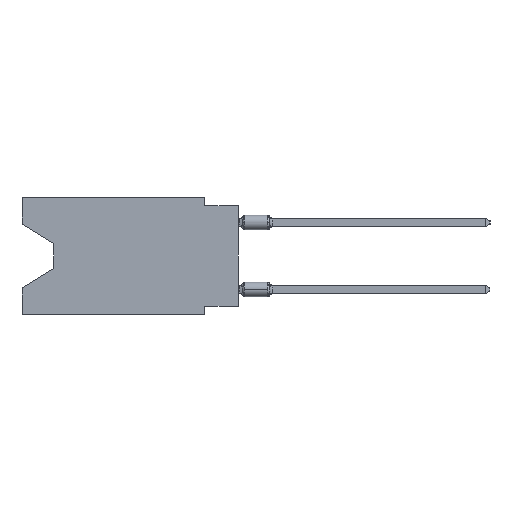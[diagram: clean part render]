
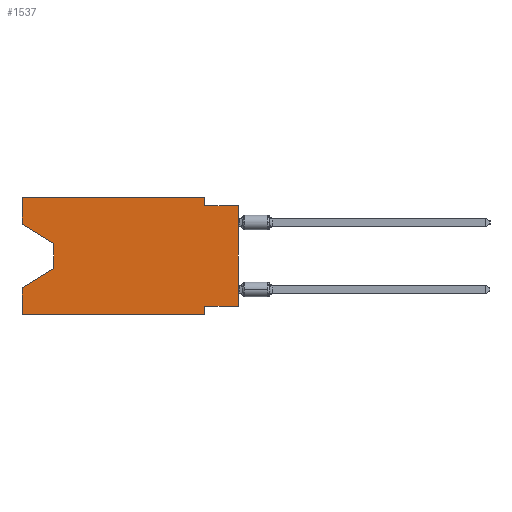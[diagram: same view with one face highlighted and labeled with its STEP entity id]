
A CAD part, left-side view. The second image highlights one B-rep face of the part: STEP entity #1537.
In plain terms, the highlighted planar face has unit normal (-1, 0, 0).
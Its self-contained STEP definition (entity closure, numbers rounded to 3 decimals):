
#347 = CARTESIAN_POINT ( 'NONE',  ( 0., 16.383, -6.852 ) ) ;
#589 = EDGE_CURVE ( 'NONE', #2754, #10713, #4848, .T. ) ;
#617 = LINE ( 'NONE', #11900, #15116 ) ;
#751 = ORIENTED_EDGE ( 'NONE', *, *, #9387, .F. ) ;
#971 = ORIENTED_EDGE ( 'NONE', *, *, #14238, .F. ) ;
#1141 = DIRECTION ( 'NONE',  ( 0., 0., -1. ) ) ;
#1215 = CARTESIAN_POINT ( 'NONE',  ( 0., 0., 0. ) ) ;
#1287 = VERTEX_POINT ( 'NONE', #16835 ) ;
#1289 = EDGE_CURVE ( 'NONE', #13922, #15580, #4266, .T. ) ;
#1366 = DIRECTION ( 'NONE',  ( 0., 0., 1. ) ) ;
#1431 = LINE ( 'NONE', #13906, #12771 ) ;
#1537 = ADVANCED_FACE ( 'NONE', ( #4064 ), #15334, .F. ) ;
#2052 = VERTEX_POINT ( 'NONE', #15244 ) ;
#2508 = DIRECTION ( 'NONE',  ( 1., 0., 0. ) ) ;
#2754 = VERTEX_POINT ( 'NONE', #2794 ) ;
#2779 = CARTESIAN_POINT ( 'NONE',  ( 0., 0., -8.255 ) ) ;
#2794 = CARTESIAN_POINT ( 'NONE',  ( 0., 16.383, -2.038 ) ) ;
#3240 = ORIENTED_EDGE ( 'NONE', *, *, #13614, .F. ) ;
#3389 = DIRECTION ( 'NONE',  ( 0., -0.855, -0.519 ) ) ;
#3928 = CARTESIAN_POINT ( 'NONE',  ( 0., 0., -0.635 ) ) ;
#3960 = EDGE_CURVE ( 'NONE', #15157, #2052, #4285, .T. ) ;
#4064 = FACE_OUTER_BOUND ( 'NONE', #15612, .T. ) ;
#4266 = LINE ( 'NONE', #8523, #13987 ) ;
#4282 = ORIENTED_EDGE ( 'NONE', *, *, #3960, .T. ) ;
#4285 = LINE ( 'NONE', #6686, #15832 ) ;
#4326 = EDGE_CURVE ( 'NONE', #4957, #5378, #617, .T. ) ;
#4848 = LINE ( 'NONE', #11570, #14271 ) ;
#4957 = VERTEX_POINT ( 'NONE', #15312 ) ;
#5256 = LINE ( 'NONE', #11119, #18089 ) ;
#5370 = ORIENTED_EDGE ( 'NONE', *, *, #11803, .T. ) ;
#5378 = VERTEX_POINT ( 'NONE', #15485 ) ;
#5820 = VECTOR ( 'NONE', #10855, 1000. ) ;
#6329 = LINE ( 'NONE', #10725, #6870 ) ;
#6411 = LINE ( 'NONE', #13378, #13973 ) ;
#6468 = EDGE_CURVE ( 'NONE', #2754, #4957, #6411, .T. ) ;
#6572 = ORIENTED_EDGE ( 'NONE', *, *, #4326, .F. ) ;
#6667 = VERTEX_POINT ( 'NONE', #15100 ) ;
#6686 = CARTESIAN_POINT ( 'NONE',  ( 0., 16.383, -8.89 ) ) ;
#6870 = VECTOR ( 'NONE', #17797, 1000. ) ;
#7025 = VERTEX_POINT ( 'NONE', #7167 ) ;
#7167 = CARTESIAN_POINT ( 'NONE',  ( 0., 13.97, -5.385 ) ) ;
#7787 = DIRECTION ( 'NONE',  ( 0., 0., 1. ) ) ;
#7943 = VERTEX_POINT ( 'NONE', #347 ) ;
#8100 = DIRECTION ( 'NONE',  ( 0., 0., -1. ) ) ;
#8456 = CARTESIAN_POINT ( 'NONE',  ( 0., 16.383, 0. ) ) ;
#8523 = CARTESIAN_POINT ( 'NONE',  ( 0., 0., -0.635 ) ) ;
#8542 = ORIENTED_EDGE ( 'NONE', *, *, #13166, .T. ) ;
#9116 = ORIENTED_EDGE ( 'NONE', *, *, #1289, .F. ) ;
#9387 = EDGE_CURVE ( 'NONE', #5378, #13922, #1431, .T. ) ;
#10087 = VECTOR ( 'NONE', #12601, 1000. ) ;
#10713 = VERTEX_POINT ( 'NONE', #15892 ) ;
#10725 = CARTESIAN_POINT ( 'NONE',  ( 0., 2.54, -8.89 ) ) ;
#10830 = EDGE_CURVE ( 'NONE', #10713, #7025, #5256, .T. ) ;
#10855 = DIRECTION ( 'NONE',  ( 0., 0., 1. ) ) ;
#11119 = CARTESIAN_POINT ( 'NONE',  ( 0., 13.97, -3.505 ) ) ;
#11570 = CARTESIAN_POINT ( 'NONE',  ( 0., 16.383, -2.038 ) ) ;
#11803 = EDGE_CURVE ( 'NONE', #7025, #7943, #12788, .T. ) ;
#11900 = CARTESIAN_POINT ( 'NONE',  ( 0., 16.383, 0. ) ) ;
#12400 = CARTESIAN_POINT ( 'NONE',  ( 0., 16.383, -8.89 ) ) ;
#12601 = DIRECTION ( 'NONE',  ( 0., 1., 0. ) ) ;
#12771 = VECTOR ( 'NONE', #18028, 1000. ) ;
#12788 = LINE ( 'NONE', #15813, #13724 ) ;
#13166 = EDGE_CURVE ( 'NONE', #6667, #15580, #13793, .T. ) ;
#13311 = VECTOR ( 'NONE', #1366, 1000. ) ;
#13372 = EDGE_CURVE ( 'NONE', #15157, #7943, #13765, .T. ) ;
#13378 = CARTESIAN_POINT ( 'NONE',  ( 0., 16.383, 0. ) ) ;
#13614 = EDGE_CURVE ( 'NONE', #6667, #1287, #18013, .T. ) ;
#13724 = VECTOR ( 'NONE', #17289, 1000. ) ;
#13765 = LINE ( 'NONE', #8456, #13311 ) ;
#13793 = LINE ( 'NONE', #1215, #5820 ) ;
#13837 = DIRECTION ( 'NONE',  ( 0., -1., 0. ) ) ;
#13885 = CARTESIAN_POINT ( 'NONE',  ( 0., 16.383, 0. ) ) ;
#13906 = CARTESIAN_POINT ( 'NONE',  ( 0., 2.54, 0. ) ) ;
#13922 = VERTEX_POINT ( 'NONE', #15318 ) ;
#13973 = VECTOR ( 'NONE', #7787, 1000. ) ;
#13987 = VECTOR ( 'NONE', #14102, 1000. ) ;
#14102 = DIRECTION ( 'NONE',  ( 0., -1., 0. ) ) ;
#14238 = EDGE_CURVE ( 'NONE', #1287, #2052, #6329, .T. ) ;
#14271 = VECTOR ( 'NONE', #3389, 1000. ) ;
#15100 = CARTESIAN_POINT ( 'NONE',  ( 0., 0., -8.255 ) ) ;
#15116 = VECTOR ( 'NONE', #16110, 1000. ) ;
#15157 = VERTEX_POINT ( 'NONE', #12400 ) ;
#15244 = CARTESIAN_POINT ( 'NONE',  ( 0., 2.54, -8.89 ) ) ;
#15312 = CARTESIAN_POINT ( 'NONE',  ( 0., 16.383, 0. ) ) ;
#15318 = CARTESIAN_POINT ( 'NONE',  ( 0., 2.54, -0.635 ) ) ;
#15334 = PLANE ( 'NONE',  #16635 ) ;
#15485 = CARTESIAN_POINT ( 'NONE',  ( 0., 2.54, 0. ) ) ;
#15580 = VERTEX_POINT ( 'NONE', #3928 ) ;
#15612 = EDGE_LOOP ( 'NONE', ( #15778, #15970, #5370, #17174, #4282, #971, #3240, #8542, #9116, #751, #6572, #16280 ) ) ;
#15778 = ORIENTED_EDGE ( 'NONE', *, *, #589, .T. ) ;
#15813 = CARTESIAN_POINT ( 'NONE',  ( 0., 13.97, -5.385 ) ) ;
#15832 = VECTOR ( 'NONE', #13837, 1000. ) ;
#15892 = CARTESIAN_POINT ( 'NONE',  ( 0., 13.97, -3.505 ) ) ;
#15970 = ORIENTED_EDGE ( 'NONE', *, *, #10830, .T. ) ;
#16110 = DIRECTION ( 'NONE',  ( 0., -1., 0. ) ) ;
#16280 = ORIENTED_EDGE ( 'NONE', *, *, #6468, .F. ) ;
#16635 = AXIS2_PLACEMENT_3D ( 'NONE', #13885, #2508, #1141 ) ;
#16835 = CARTESIAN_POINT ( 'NONE',  ( 0., 2.54, -8.255 ) ) ;
#17174 = ORIENTED_EDGE ( 'NONE', *, *, #13372, .F. ) ;
#17289 = DIRECTION ( 'NONE',  ( 0., 0.855, -0.519 ) ) ;
#17797 = DIRECTION ( 'NONE',  ( 0., 0., -1. ) ) ;
#18013 = LINE ( 'NONE', #2779, #10087 ) ;
#18028 = DIRECTION ( 'NONE',  ( 0., 0., -1. ) ) ;
#18089 = VECTOR ( 'NONE', #8100, 1000. ) ;
